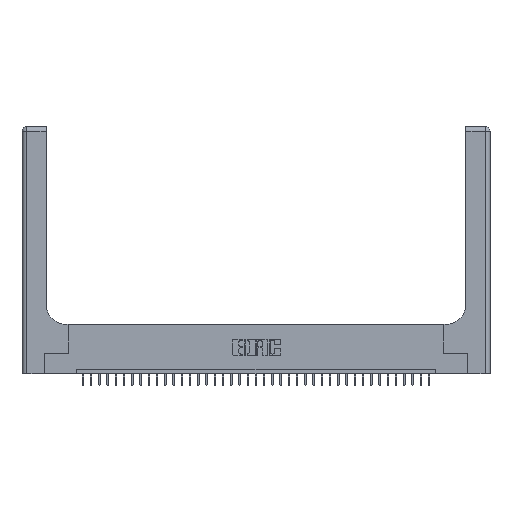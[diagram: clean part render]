
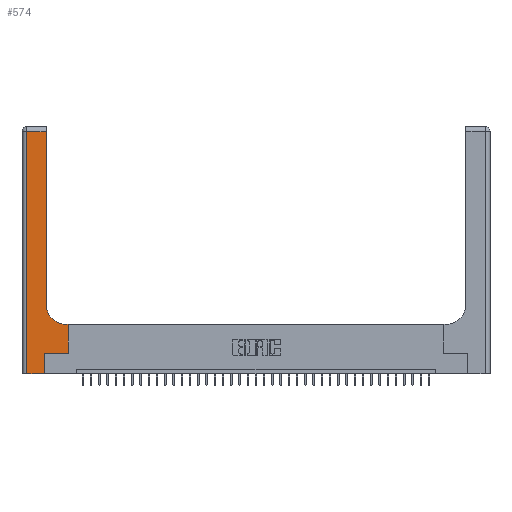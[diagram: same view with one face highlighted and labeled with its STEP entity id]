
A CAD part, top view. The second image highlights one B-rep face of the part: STEP entity #574.
In plain terms, the highlighted planar face has unit normal (0, 0, 1).
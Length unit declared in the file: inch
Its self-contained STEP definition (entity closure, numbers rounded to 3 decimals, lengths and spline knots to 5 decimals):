
#176 = PLANE ( 'NONE',  #24144 ) ;
#202 = CARTESIAN_POINT ( 'NONE',  ( 0.06, 2.94, 0.37 ) ) ;
#574 = ADVANCED_FACE ( 'NONE', ( #17260 ), #176, .F. ) ;
#2030 = LINE ( 'NONE', #31258, #15426 ) ;
#3400 = DIRECTION ( 'NONE',  ( 1., 0., 0. ) ) ;
#3958 = CIRCLE ( 'NONE', #13655, 0.25 ) ;
#4331 = EDGE_LOOP ( 'NONE', ( #18572, #18418, #12394, #32865, #29305, #26431, #28789, #28244, #4805 ) ) ;
#4805 = ORIENTED_EDGE ( 'NONE', *, *, #23763, .T. ) ;
#6665 = VECTOR ( 'NONE', #3400, 39.37008 ) ;
#6883 = DIRECTION ( 'NONE',  ( 1., 0., 0. ) ) ;
#6989 = LINE ( 'NONE', #15106, #36284 ) ;
#7155 = DIRECTION ( 'NONE',  ( 0., -1., 0. ) ) ;
#8541 = CARTESIAN_POINT ( 'NONE',  ( 0., 3., 0.37 ) ) ;
#8697 = VECTOR ( 'NONE', #12545, 39.37008 ) ;
#9114 = EDGE_CURVE ( 'NONE', #25403, #30996, #36963, .T. ) ;
#9886 = CARTESIAN_POINT ( 'NONE',  ( 0.5415, 0.85, 0.37 ) ) ;
#10190 = CARTESIAN_POINT ( 'NONE',  ( 0.269, 0.25, 0.37 ) ) ;
#10191 = EDGE_CURVE ( 'NONE', #17158, #25403, #29384, .T. ) ;
#11038 = CARTESIAN_POINT ( 'NONE',  ( 0., 0., 0.37 ) ) ;
#11107 = CARTESIAN_POINT ( 'NONE',  ( 0., 2.94, 0.37 ) ) ;
#11362 = VERTEX_POINT ( 'NONE', #32045 ) ;
#11478 = CARTESIAN_POINT ( 'NONE',  ( 0.2915, 3., 0.37 ) ) ;
#11527 = VECTOR ( 'NONE', #34466, 39.37008 ) ;
#11744 = VERTEX_POINT ( 'NONE', #34110 ) ;
#11924 = DIRECTION ( 'NONE',  ( -1., 0., 0. ) ) ;
#11978 = LINE ( 'NONE', #24115, #30826 ) ;
#12394 = ORIENTED_EDGE ( 'NONE', *, *, #12636, .T. ) ;
#12395 = VECTOR ( 'NONE', #36748, 39.37008 ) ;
#12545 = DIRECTION ( 'NONE',  ( -1., 0., 0. ) ) ;
#12636 = EDGE_CURVE ( 'NONE', #30433, #17158, #6989, .T. ) ;
#12676 = CARTESIAN_POINT ( 'NONE',  ( 0.5585, 0.6, 0.37 ) ) ;
#13298 = DIRECTION ( 'NONE',  ( 1., 0., 0. ) ) ;
#13655 = AXIS2_PLACEMENT_3D ( 'NONE', #9886, #30186, #13298 ) ;
#14975 = EDGE_CURVE ( 'NONE', #11362, #21877, #28949, .T. ) ;
#15106 = CARTESIAN_POINT ( 'NONE',  ( 0.06, 3., 0.37 ) ) ;
#15165 = CARTESIAN_POINT ( 'NONE',  ( 0.06, 0., 0.37 ) ) ;
#15426 = VECTOR ( 'NONE', #37123, 39.37008 ) ;
#16245 = VERTEX_POINT ( 'NONE', #20039 ) ;
#16643 = CARTESIAN_POINT ( 'NONE',  ( 0.269, 0., 0.37 ) ) ;
#17158 = VERTEX_POINT ( 'NONE', #15165 ) ;
#17260 = FACE_OUTER_BOUND ( 'NONE', #4331, .T. ) ;
#18418 = ORIENTED_EDGE ( 'NONE', *, *, #35105, .T. ) ;
#18572 = ORIENTED_EDGE ( 'NONE', *, *, #14975, .T. ) ;
#19320 = CARTESIAN_POINT ( 'NONE',  ( 0.269, 0., 0.37 ) ) ;
#20039 = CARTESIAN_POINT ( 'NONE',  ( 0.5415, 0.6, 0.37 ) ) ;
#21877 = VERTEX_POINT ( 'NONE', #36107 ) ;
#23139 = DIRECTION ( 'NONE',  ( 0., 0., -1. ) ) ;
#23763 = EDGE_CURVE ( 'NONE', #16245, #11362, #3958, .T. ) ;
#24115 = CARTESIAN_POINT ( 'NONE',  ( 0.269, 0.25, 0.37 ) ) ;
#24144 = AXIS2_PLACEMENT_3D ( 'NONE', #8541, #23139, #11924 ) ;
#25403 = VERTEX_POINT ( 'NONE', #19320 ) ;
#25568 = DIRECTION ( 'NONE',  ( 0., 1., 0. ) ) ;
#26431 = ORIENTED_EDGE ( 'NONE', *, *, #26503, .T. ) ;
#26503 = EDGE_CURVE ( 'NONE', #30996, #11744, #11978, .T. ) ;
#27133 = LINE ( 'NONE', #29244, #8697 ) ;
#28244 = ORIENTED_EDGE ( 'NONE', *, *, #33516, .T. ) ;
#28789 = ORIENTED_EDGE ( 'NONE', *, *, #35154, .T. ) ;
#28949 = LINE ( 'NONE', #11478, #11527 ) ;
#29244 = CARTESIAN_POINT ( 'NONE',  ( 0.2915, 0.6, 0.37 ) ) ;
#29305 = ORIENTED_EDGE ( 'NONE', *, *, #9114, .T. ) ;
#29384 = LINE ( 'NONE', #11038, #6665 ) ;
#30186 = DIRECTION ( 'NONE',  ( 0., 0., -1. ) ) ;
#30433 = VERTEX_POINT ( 'NONE', #202 ) ;
#30826 = VECTOR ( 'NONE', #6883, 39.37008 ) ;
#30996 = VERTEX_POINT ( 'NONE', #10190 ) ;
#31258 = CARTESIAN_POINT ( 'NONE',  ( 0.5585, 0.25, 0.37 ) ) ;
#32045 = CARTESIAN_POINT ( 'NONE',  ( 0.2915, 0.85, 0.37 ) ) ;
#32173 = VERTEX_POINT ( 'NONE', #12676 ) ;
#32865 = ORIENTED_EDGE ( 'NONE', *, *, #10191, .T. ) ;
#33516 = EDGE_CURVE ( 'NONE', #32173, #16245, #27133, .T. ) ;
#33697 = VECTOR ( 'NONE', #25568, 39.37008 ) ;
#34110 = CARTESIAN_POINT ( 'NONE',  ( 0.5585, 0.25, 0.37 ) ) ;
#34277 = LINE ( 'NONE', #11107, #12395 ) ;
#34466 = DIRECTION ( 'NONE',  ( 0., 1., 0. ) ) ;
#35105 = EDGE_CURVE ( 'NONE', #21877, #30433, #34277, .T. ) ;
#35154 = EDGE_CURVE ( 'NONE', #11744, #32173, #2030, .T. ) ;
#36107 = CARTESIAN_POINT ( 'NONE',  ( 0.2915, 2.94, 0.37 ) ) ;
#36284 = VECTOR ( 'NONE', #7155, 39.37008 ) ;
#36748 = DIRECTION ( 'NONE',  ( -1., 0., 0. ) ) ;
#36963 = LINE ( 'NONE', #16643, #33697 ) ;
#37123 = DIRECTION ( 'NONE',  ( 0., 1., 0. ) ) ;
